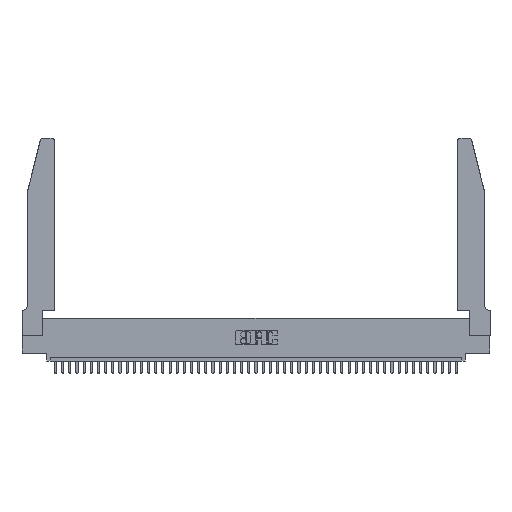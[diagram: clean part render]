
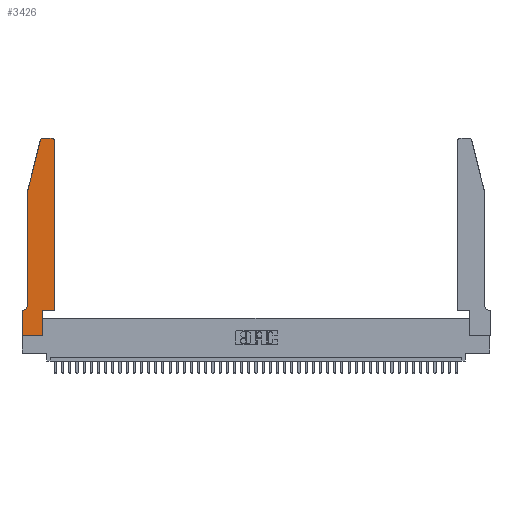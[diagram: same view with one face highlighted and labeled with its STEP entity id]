
A CAD part, top view. The second image highlights one B-rep face of the part: STEP entity #3426.
In plain terms, the highlighted planar face has unit normal (0, 0, 1).
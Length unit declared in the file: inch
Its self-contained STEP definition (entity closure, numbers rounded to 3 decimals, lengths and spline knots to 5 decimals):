
#262 = LINE ( 'NONE', #41534, #26907 ) ;
#1009 = DIRECTION ( 'NONE',  ( -1., 0., 0. ) ) ;
#1063 = LINE ( 'NONE', #29049, #18796 ) ;
#1731 = LINE ( 'NONE', #6833, #7854 ) ;
#2795 = CARTESIAN_POINT ( 'NONE',  ( 0.4505, 0.35, 0.37 ) ) ;
#2830 = VECTOR ( 'NONE', #4041, 39.37008 ) ;
#3090 = CARTESIAN_POINT ( 'NONE',  ( 0.25487, 2.72718, 0.37 ) ) ;
#3426 = ADVANCED_FACE ( 'NONE', ( #12604 ), #28938, .T. ) ;
#4041 = DIRECTION ( 'NONE',  ( 1., 0., 0. ) ) ;
#4140 = CARTESIAN_POINT ( 'NONE',  ( 0., 0.35, 0.37 ) ) ;
#4782 = VERTEX_POINT ( 'NONE', #8969 ) ;
#5052 = CIRCLE ( 'NONE', #17598, 0.03 ) ;
#5712 = CARTESIAN_POINT ( 'NONE',  ( 0., 0., 0.37 ) ) ;
#6595 = DIRECTION ( 'NONE',  ( -1., 0., 0. ) ) ;
#6833 = CARTESIAN_POINT ( 'NONE',  ( 0.4505, 0.35, 0.37 ) ) ;
#6983 = EDGE_CURVE ( 'NONE', #4782, #41300, #5052, .T. ) ;
#7712 = DIRECTION ( 'NONE',  ( 0., 0., 1. ) ) ;
#7780 = LINE ( 'NONE', #5712, #8906 ) ;
#7854 = VECTOR ( 'NONE', #21760, 39.37008 ) ;
#8298 = AXIS2_PLACEMENT_3D ( 'NONE', #4140, #7712, #11222 ) ;
#8464 = CARTESIAN_POINT ( 'NONE',  ( 0.284, 2.75, 0.37 ) ) ;
#8906 = VECTOR ( 'NONE', #9075, 39.37008 ) ;
#8969 = CARTESIAN_POINT ( 'NONE',  ( 0.4505, 2.72, 0.37 ) ) ;
#8983 = VERTEX_POINT ( 'NONE', #14730 ) ;
#9075 = DIRECTION ( 'NONE',  ( 1., 0., 0. ) ) ;
#10082 = VECTOR ( 'NONE', #39893, 39.37008 ) ;
#10383 = ORIENTED_EDGE ( 'NONE', *, *, #40753, .T. ) ;
#11222 = DIRECTION ( 'NONE',  ( 1., 0., 0. ) ) ;
#11410 = CARTESIAN_POINT ( 'NONE',  ( 0.0755, 2., 0.37 ) ) ;
#11469 = DIRECTION ( 'NONE',  ( -1., 0., 0. ) ) ;
#11656 = EDGE_CURVE ( 'NONE', #35748, #22441, #7780, .T. ) ;
#11797 = VERTEX_POINT ( 'NONE', #37739 ) ;
#12217 = LINE ( 'NONE', #42775, #2830 ) ;
#12604 = FACE_OUTER_BOUND ( 'NONE', #24736, .T. ) ;
#12775 = EDGE_CURVE ( 'NONE', #14945, #28318, #43156, .T. ) ;
#13848 = CIRCLE ( 'NONE', #36371, 0.07 ) ;
#13949 = DIRECTION ( 'NONE',  ( 0., 0., 1. ) ) ;
#13954 = VERTEX_POINT ( 'NONE', #2795 ) ;
#14091 = DIRECTION ( 'NONE',  ( 1., 0., 0. ) ) ;
#14730 = CARTESIAN_POINT ( 'NONE',  ( 0., 0.35, 0.37 ) ) ;
#14797 = AXIS2_PLACEMENT_3D ( 'NONE', #24702, #21809, #36063 ) ;
#14945 = VERTEX_POINT ( 'NONE', #8464 ) ;
#15594 = ORIENTED_EDGE ( 'NONE', *, *, #11656, .T. ) ;
#15852 = CARTESIAN_POINT ( 'NONE',  ( 0.4205, 2.75, 0.37 ) ) ;
#17353 = LINE ( 'NONE', #26091, #34591 ) ;
#17516 = ORIENTED_EDGE ( 'NONE', *, *, #17664, .T. ) ;
#17598 = AXIS2_PLACEMENT_3D ( 'NONE', #27824, #13949, #14091 ) ;
#17664 = EDGE_CURVE ( 'NONE', #32468, #17957, #31200, .T. ) ;
#17858 = ORIENTED_EDGE ( 'NONE', *, *, #24149, .T. ) ;
#17957 = VERTEX_POINT ( 'NONE', #29556 ) ;
#17963 = CARTESIAN_POINT ( 'NONE',  ( 0.2865, 0., 0.37 ) ) ;
#18327 = DIRECTION ( 'NONE',  ( 0., 1., 0. ) ) ;
#18796 = VECTOR ( 'NONE', #18327, 39.37008 ) ;
#20405 = VECTOR ( 'NONE', #29904, 39.37008 ) ;
#20468 = DIRECTION ( 'NONE',  ( 0., -1., 0. ) ) ;
#20888 = ORIENTED_EDGE ( 'NONE', *, *, #44327, .T. ) ;
#20909 = CARTESIAN_POINT ( 'NONE',  ( 0.0055, 0.35, 0.37 ) ) ;
#21760 = DIRECTION ( 'NONE',  ( 0., 1., 0. ) ) ;
#21809 = DIRECTION ( 'NONE',  ( 0., 0., 1. ) ) ;
#21946 = ORIENTED_EDGE ( 'NONE', *, *, #35328, .T. ) ;
#22142 = ORIENTED_EDGE ( 'NONE', *, *, #28021, .T. ) ;
#22232 = CARTESIAN_POINT ( 'NONE',  ( 0.0055, 0.42, 0.37 ) ) ;
#22441 = VERTEX_POINT ( 'NONE', #17963 ) ;
#22849 = LINE ( 'NONE', #34786, #25554 ) ;
#24149 = EDGE_CURVE ( 'NONE', #13954, #4782, #1731, .T. ) ;
#24236 = EDGE_CURVE ( 'NONE', #29027, #8983, #22849, .T. ) ;
#24702 = CARTESIAN_POINT ( 'NONE',  ( 0.284, 2.72, 0.37 ) ) ;
#24736 = EDGE_LOOP ( 'NONE', ( #40909, #45834, #21946, #17516, #22142, #43431, #10383, #15594, #20888, #30412, #17858, #43375 ) ) ;
#25554 = VECTOR ( 'NONE', #6595, 39.37008 ) ;
#26091 = CARTESIAN_POINT ( 'NONE',  ( 0.2605, 2.75, 0.37 ) ) ;
#26360 = CARTESIAN_POINT ( 'NONE',  ( 0.0755, 2., 0.37 ) ) ;
#26907 = VECTOR ( 'NONE', #20468, 39.37008 ) ;
#27824 = CARTESIAN_POINT ( 'NONE',  ( 0.4205, 2.72, 0.37 ) ) ;
#28021 = EDGE_CURVE ( 'NONE', #17957, #29027, #13848, .T. ) ;
#28182 = EDGE_CURVE ( 'NONE', #11797, #13954, #12217, .T. ) ;
#28318 = VERTEX_POINT ( 'NONE', #3090 ) ;
#28938 = PLANE ( 'NONE',  #8298 ) ;
#29027 = VERTEX_POINT ( 'NONE', #20909 ) ;
#29049 = CARTESIAN_POINT ( 'NONE',  ( 0.2865, 0.35, 0.37 ) ) ;
#29556 = CARTESIAN_POINT ( 'NONE',  ( 0.0755, 0.42, 0.37 ) ) ;
#29904 = DIRECTION ( 'NONE',  ( -0.239, -0.971, 0. ) ) ;
#30412 = ORIENTED_EDGE ( 'NONE', *, *, #28182, .T. ) ;
#31010 = CARTESIAN_POINT ( 'NONE',  ( 0.0755, 2., 0.37 ) ) ;
#31200 = LINE ( 'NONE', #11410, #10082 ) ;
#32468 = VERTEX_POINT ( 'NONE', #31010 ) ;
#32590 = EDGE_CURVE ( 'NONE', #41300, #14945, #17353, .T. ) ;
#34591 = VECTOR ( 'NONE', #11469, 39.37008 ) ;
#34786 = CARTESIAN_POINT ( 'NONE',  ( 0.0755, 0.35, 0.37 ) ) ;
#35328 = EDGE_CURVE ( 'NONE', #28318, #32468, #35394, .T. ) ;
#35394 = LINE ( 'NONE', #26360, #20405 ) ;
#35748 = VERTEX_POINT ( 'NONE', #43804 ) ;
#36063 = DIRECTION ( 'NONE',  ( 1., 0., 0. ) ) ;
#36371 = AXIS2_PLACEMENT_3D ( 'NONE', #22232, #36801, #1009 ) ;
#36801 = DIRECTION ( 'NONE',  ( 0., 0., -1. ) ) ;
#37739 = CARTESIAN_POINT ( 'NONE',  ( 0.2865, 0.35, 0.37 ) ) ;
#39893 = DIRECTION ( 'NONE',  ( 0., -1., 0. ) ) ;
#40753 = EDGE_CURVE ( 'NONE', #8983, #35748, #262, .T. ) ;
#40909 = ORIENTED_EDGE ( 'NONE', *, *, #32590, .T. ) ;
#41300 = VERTEX_POINT ( 'NONE', #15852 ) ;
#41534 = CARTESIAN_POINT ( 'NONE',  ( 0., 0., 0.37 ) ) ;
#42775 = CARTESIAN_POINT ( 'NONE',  ( 0.4505, 0.35, 0.37 ) ) ;
#43156 = CIRCLE ( 'NONE', #14797, 0.03 ) ;
#43375 = ORIENTED_EDGE ( 'NONE', *, *, #6983, .T. ) ;
#43431 = ORIENTED_EDGE ( 'NONE', *, *, #24236, .T. ) ;
#43804 = CARTESIAN_POINT ( 'NONE',  ( 0., 0., 0.37 ) ) ;
#44327 = EDGE_CURVE ( 'NONE', #22441, #11797, #1063, .T. ) ;
#45834 = ORIENTED_EDGE ( 'NONE', *, *, #12775, .T. ) ;
